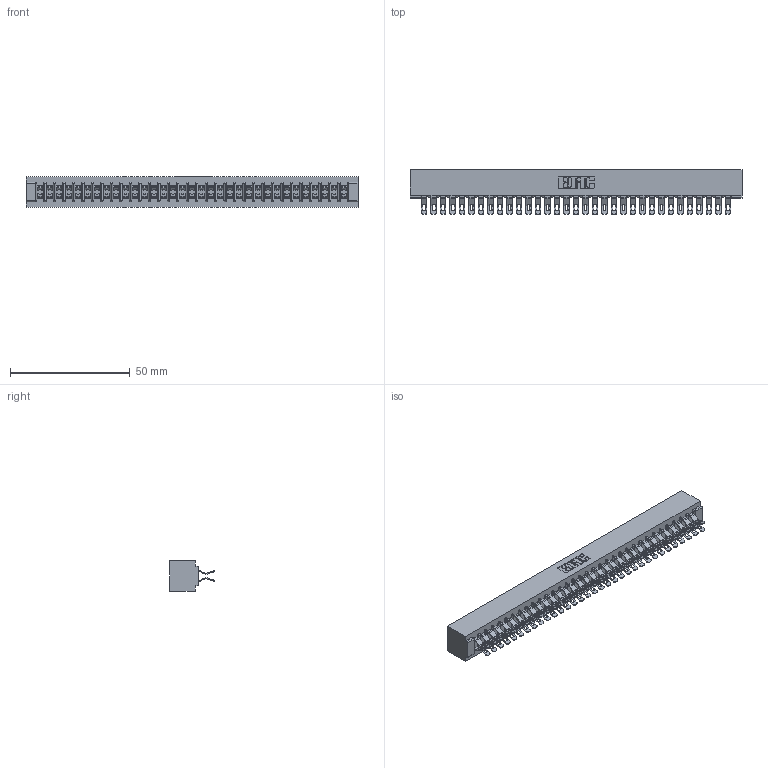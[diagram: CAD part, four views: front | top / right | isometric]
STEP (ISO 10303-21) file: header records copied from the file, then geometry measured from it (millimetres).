
FILE_DESCRIPTION (( 'STEP AP203' ), '1' );
FILE_NAME ('357-066-555-201.STEP', '2018-08-12T17:19:05', ( '' ), ( '' ), 'SwSTEP 2.0', 'SolidWorks 2016', '' );
FILE_SCHEMA (( 'CONFIG_CONTROL_DESIGN' ));
Length unit declared in the file: inch
Products named in the file (3): 307 Part_No Mounting Lugs; 307-290-001_555; 357-066-555-201
Assembly tree (67 placements, depth 2):
  357-066-555-201
    307 Part_No Mounting Lugs
    307-290-001_555  x66
Bounding box: 138.63 x 18.75 x 12.7 mm (x, y, z)
Volume: 15422.4 mm3; surface area: 20094.9 mm2
Topology: 67 solids, 67 shells, 4170 faces, 12245 edges, 7982 vertices
Faces by surface type: plane 2310, cylinder 1792, sphere 68
Entity records: 30715 total; most frequent: CARTESIAN_POINT 5029, ORIENTED_EDGE 4984, DIRECTION 4936, EDGE_CURVE 2492, LINE 1898, VECTOR 1898, VERTEX_POINT 1612, AXIS2_PLACEMENT_3D 1519
